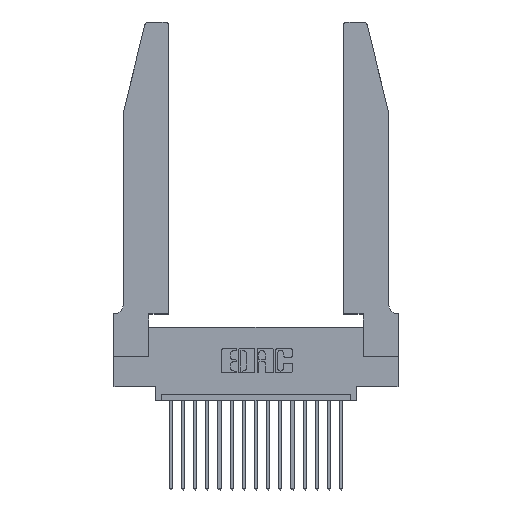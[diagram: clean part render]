
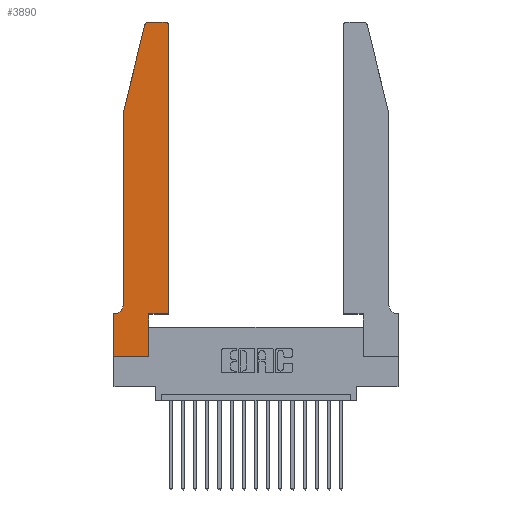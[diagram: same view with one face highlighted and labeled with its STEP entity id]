
A CAD part, top view. The second image highlights one B-rep face of the part: STEP entity #3890.
In plain terms, the highlighted planar face has unit normal (0, 0, 1).
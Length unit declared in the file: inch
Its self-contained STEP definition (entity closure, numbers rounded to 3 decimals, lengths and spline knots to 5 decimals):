
#269 = CARTESIAN_POINT ( 'NONE',  ( 0., 0., 0.37 ) ) ;
#604 = FACE_OUTER_BOUND ( 'NONE', #12123, .T. ) ;
#701 = VERTEX_POINT ( 'NONE', #17620 ) ;
#962 = DIRECTION ( 'NONE',  ( 1., 0., 0. ) ) ;
#1764 = CARTESIAN_POINT ( 'NONE',  ( 0., 0.35, 0.37 ) ) ;
#2481 = DIRECTION ( 'NONE',  ( 0., -1., 0. ) ) ;
#2589 = CARTESIAN_POINT ( 'NONE',  ( 0.4505, 0.35, 0.37 ) ) ;
#2696 = ORIENTED_EDGE ( 'NONE', *, *, #16956, .T. ) ;
#2924 = DIRECTION ( 'NONE',  ( 1., 0., 0. ) ) ;
#2978 = ORIENTED_EDGE ( 'NONE', *, *, #6064, .T. ) ;
#2990 = VECTOR ( 'NONE', #2481, 39.37008 ) ;
#3202 = EDGE_CURVE ( 'NONE', #3948, #701, #19357, .T. ) ;
#3519 = VERTEX_POINT ( 'NONE', #8728 ) ;
#3726 = LINE ( 'NONE', #9826, #2990 ) ;
#3763 = LINE ( 'NONE', #269, #16648 ) ;
#3890 = ADVANCED_FACE ( 'NONE', ( #604 ), #10820, .T. ) ;
#3948 = VERTEX_POINT ( 'NONE', #12026 ) ;
#3994 = LINE ( 'NONE', #16050, #11381 ) ;
#4115 = EDGE_CURVE ( 'NONE', #15553, #5860, #3994, .T. ) ;
#4427 = CIRCLE ( 'NONE', #12927, 0.03 ) ;
#4527 = CARTESIAN_POINT ( 'NONE',  ( 0.2865, 0.35, 0.37 ) ) ;
#4721 = DIRECTION ( 'NONE',  ( -1., 0., 0. ) ) ;
#5265 = DIRECTION ( 'NONE',  ( 0., 0., -1. ) ) ;
#5622 = EDGE_CURVE ( 'NONE', #701, #16446, #3726, .T. ) ;
#5711 = CARTESIAN_POINT ( 'NONE',  ( 0.0055, 0.35, 0.37 ) ) ;
#5860 = VERTEX_POINT ( 'NONE', #13822 ) ;
#6064 = EDGE_CURVE ( 'NONE', #15240, #10221, #16808, .T. ) ;
#6424 = CIRCLE ( 'NONE', #12716, 0.07 ) ;
#6532 = CARTESIAN_POINT ( 'NONE',  ( 0.2865, 0.35, 0.37 ) ) ;
#6625 = CARTESIAN_POINT ( 'NONE',  ( 0.4505, 2.72, 0.37 ) ) ;
#6816 = EDGE_CURVE ( 'NONE', #17089, #3519, #10328, .T. ) ;
#6930 = DIRECTION ( 'NONE',  ( 0., -1., 0. ) ) ;
#6972 = CARTESIAN_POINT ( 'NONE',  ( 0.0055, 0.42, 0.37 ) ) ;
#7024 = VERTEX_POINT ( 'NONE', #5711 ) ;
#7235 = ORIENTED_EDGE ( 'NONE', *, *, #4115, .T. ) ;
#7620 = AXIS2_PLACEMENT_3D ( 'NONE', #9813, #15792, #14533 ) ;
#7744 = CARTESIAN_POINT ( 'NONE',  ( 0.4505, 0.35, 0.37 ) ) ;
#7786 = DIRECTION ( 'NONE',  ( 0., 0., 1. ) ) ;
#7925 = ORIENTED_EDGE ( 'NONE', *, *, #17837, .T. ) ;
#7961 = EDGE_CURVE ( 'NONE', #7024, #15553, #12436, .T. ) ;
#7967 = VECTOR ( 'NONE', #19286, 39.37008 ) ;
#8728 = CARTESIAN_POINT ( 'NONE',  ( 0.4205, 2.75, 0.37 ) ) ;
#9360 = ORIENTED_EDGE ( 'NONE', *, *, #16383, .T. ) ;
#9671 = DIRECTION ( 'NONE',  ( 1., 0., 0. ) ) ;
#9813 = CARTESIAN_POINT ( 'NONE',  ( 0., 0.35, 0.37 ) ) ;
#9826 = CARTESIAN_POINT ( 'NONE',  ( 0.0755, 2., 0.37 ) ) ;
#10221 = VERTEX_POINT ( 'NONE', #4527 ) ;
#10328 = CIRCLE ( 'NONE', #14700, 0.03 ) ;
#10354 = CARTESIAN_POINT ( 'NONE',  ( 0.0755, 0.35, 0.37 ) ) ;
#10595 = ORIENTED_EDGE ( 'NONE', *, *, #17943, .T. ) ;
#10599 = ORIENTED_EDGE ( 'NONE', *, *, #6816, .T. ) ;
#10652 = DIRECTION ( 'NONE',  ( 1., 0., 0. ) ) ;
#10723 = EDGE_CURVE ( 'NONE', #5860, #15240, #3763, .T. ) ;
#10820 = PLANE ( 'NONE',  #7620 ) ;
#10923 = VECTOR ( 'NONE', #9671, 39.37008 ) ;
#11381 = VECTOR ( 'NONE', #6930, 39.37008 ) ;
#12026 = CARTESIAN_POINT ( 'NONE',  ( 0.25487, 2.72718, 0.37 ) ) ;
#12123 = EDGE_LOOP ( 'NONE', ( #10595, #2696, #12134, #15344, #19719, #17425, #7235, #15003, #2978, #9360, #7925, #10599 ) ) ;
#12134 = ORIENTED_EDGE ( 'NONE', *, *, #3202, .T. ) ;
#12436 = LINE ( 'NONE', #10354, #14360 ) ;
#12716 = AXIS2_PLACEMENT_3D ( 'NONE', #6972, #5265, #15971 ) ;
#12835 = CARTESIAN_POINT ( 'NONE',  ( 0.4505, 0.35, 0.37 ) ) ;
#12927 = AXIS2_PLACEMENT_3D ( 'NONE', #13854, #7786, #10652 ) ;
#13089 = CARTESIAN_POINT ( 'NONE',  ( 0.4205, 2.72, 0.37 ) ) ;
#13147 = CARTESIAN_POINT ( 'NONE',  ( 0.2605, 2.75, 0.37 ) ) ;
#13747 = CARTESIAN_POINT ( 'NONE',  ( 0.284, 2.75, 0.37 ) ) ;
#13822 = CARTESIAN_POINT ( 'NONE',  ( 0., 0., 0.37 ) ) ;
#13854 = CARTESIAN_POINT ( 'NONE',  ( 0.284, 2.72, 0.37 ) ) ;
#14145 = CARTESIAN_POINT ( 'NONE',  ( 0.0755, 0.42, 0.37 ) ) ;
#14360 = VECTOR ( 'NONE', #4721, 39.37008 ) ;
#14372 = DIRECTION ( 'NONE',  ( 0., 1., 0. ) ) ;
#14446 = EDGE_CURVE ( 'NONE', #16446, #7024, #6424, .T. ) ;
#14533 = DIRECTION ( 'NONE',  ( 1., 0., 0. ) ) ;
#14626 = VERTEX_POINT ( 'NONE', #2589 ) ;
#14692 = LINE ( 'NONE', #13147, #7967 ) ;
#14700 = AXIS2_PLACEMENT_3D ( 'NONE', #13089, #16308, #962 ) ;
#15003 = ORIENTED_EDGE ( 'NONE', *, *, #10723, .T. ) ;
#15240 = VERTEX_POINT ( 'NONE', #16346 ) ;
#15344 = ORIENTED_EDGE ( 'NONE', *, *, #5622, .T. ) ;
#15553 = VERTEX_POINT ( 'NONE', #1764 ) ;
#15792 = DIRECTION ( 'NONE',  ( 0., 0., 1. ) ) ;
#15883 = VECTOR ( 'NONE', #18762, 39.37008 ) ;
#15971 = DIRECTION ( 'NONE',  ( -1., 0., 0. ) ) ;
#16050 = CARTESIAN_POINT ( 'NONE',  ( 0., 0., 0.37 ) ) ;
#16285 = VECTOR ( 'NONE', #18467, 39.37008 ) ;
#16308 = DIRECTION ( 'NONE',  ( 0., 0., 1. ) ) ;
#16346 = CARTESIAN_POINT ( 'NONE',  ( 0.2865, 0., 0.37 ) ) ;
#16383 = EDGE_CURVE ( 'NONE', #10221, #14626, #19506, .T. ) ;
#16446 = VERTEX_POINT ( 'NONE', #14145 ) ;
#16596 = LINE ( 'NONE', #12835, #19185 ) ;
#16648 = VECTOR ( 'NONE', #2924, 39.37008 ) ;
#16776 = CARTESIAN_POINT ( 'NONE',  ( 0.0755, 2., 0.37 ) ) ;
#16808 = LINE ( 'NONE', #6532, #15883 ) ;
#16956 = EDGE_CURVE ( 'NONE', #18212, #3948, #4427, .T. ) ;
#17089 = VERTEX_POINT ( 'NONE', #6625 ) ;
#17425 = ORIENTED_EDGE ( 'NONE', *, *, #7961, .T. ) ;
#17620 = CARTESIAN_POINT ( 'NONE',  ( 0.0755, 2., 0.37 ) ) ;
#17837 = EDGE_CURVE ( 'NONE', #14626, #17089, #16596, .T. ) ;
#17943 = EDGE_CURVE ( 'NONE', #3519, #18212, #14692, .T. ) ;
#18212 = VERTEX_POINT ( 'NONE', #13747 ) ;
#18467 = DIRECTION ( 'NONE',  ( -0.239, -0.971, 0. ) ) ;
#18762 = DIRECTION ( 'NONE',  ( 0., 1., 0. ) ) ;
#19185 = VECTOR ( 'NONE', #14372, 39.37008 ) ;
#19286 = DIRECTION ( 'NONE',  ( -1., 0., 0. ) ) ;
#19357 = LINE ( 'NONE', #16776, #16285 ) ;
#19506 = LINE ( 'NONE', #7744, #10923 ) ;
#19719 = ORIENTED_EDGE ( 'NONE', *, *, #14446, .T. ) ;
